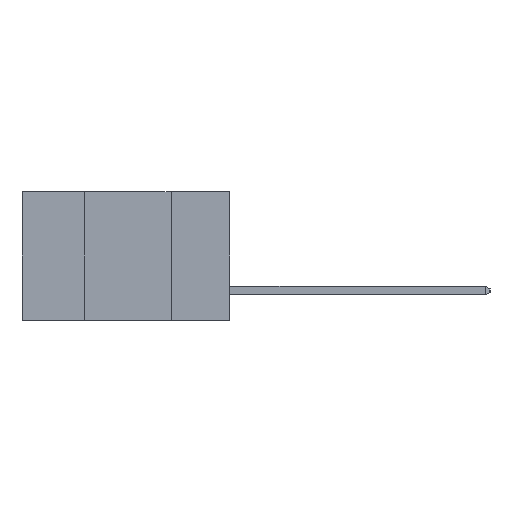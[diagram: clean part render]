
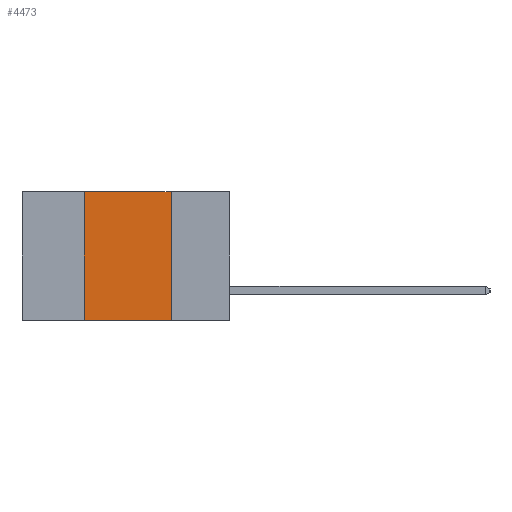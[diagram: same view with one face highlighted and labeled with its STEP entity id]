
A CAD part, left-side view. The second image highlights one B-rep face of the part: STEP entity #4473.
In plain terms, the highlighted planar face has unit normal (-1, 0, 0).
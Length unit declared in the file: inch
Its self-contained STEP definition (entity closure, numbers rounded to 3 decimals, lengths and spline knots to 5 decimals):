
#87 = CARTESIAN_POINT ( 'NONE',  ( 0., 0.6, 0. ) ) ;
#470 = DIRECTION ( 'NONE',  ( 1., 0., 0. ) ) ;
#534 = DIRECTION ( 'NONE',  ( 0., 0., -1. ) ) ;
#756 = EDGE_CURVE ( 'NONE', #3559, #2636, #8635, .T. ) ;
#881 = VERTEX_POINT ( 'NONE', #5766 ) ;
#1066 = EDGE_LOOP ( 'NONE', ( #6810, #4870, #7069, #7345 ) ) ;
#1319 = PLANE ( 'NONE',  #10908 ) ;
#1651 = CARTESIAN_POINT ( 'NONE',  ( 0., 0.17, -0.37 ) ) ;
#1844 = CARTESIAN_POINT ( 'NONE',  ( 0., 0.6, -0.37 ) ) ;
#1990 = EDGE_CURVE ( 'NONE', #881, #3559, #8235, .T. ) ;
#2378 = CARTESIAN_POINT ( 'NONE',  ( 0., 0.17, 0. ) ) ;
#2571 = CARTESIAN_POINT ( 'NONE',  ( 0., 0.6, 0. ) ) ;
#2636 = VERTEX_POINT ( 'NONE', #2378 ) ;
#2643 = CARTESIAN_POINT ( 'NONE',  ( 0., 0.17, -0.37 ) ) ;
#3559 = VERTEX_POINT ( 'NONE', #5365 ) ;
#3586 = DIRECTION ( 'NONE',  ( 0., -1., 0. ) ) ;
#4473 = ADVANCED_FACE ( 'NONE', ( #8556 ), #1319, .F. ) ;
#4870 = ORIENTED_EDGE ( 'NONE', *, *, #756, .F. ) ;
#5365 = CARTESIAN_POINT ( 'NONE',  ( 0., 0.42, 0. ) ) ;
#5766 = CARTESIAN_POINT ( 'NONE',  ( 0., 0.42, -0.37 ) ) ;
#6008 = VECTOR ( 'NONE', #7766, 39.37008 ) ;
#6066 = VERTEX_POINT ( 'NONE', #1651 ) ;
#6188 = DIRECTION ( 'NONE',  ( 0., -1., 0. ) ) ;
#6428 = VECTOR ( 'NONE', #3586, 39.37008 ) ;
#6619 = LINE ( 'NONE', #1844, #10853 ) ;
#6810 = ORIENTED_EDGE ( 'NONE', *, *, #9561, .F. ) ;
#7069 = ORIENTED_EDGE ( 'NONE', *, *, #1990, .F. ) ;
#7345 = ORIENTED_EDGE ( 'NONE', *, *, #9023, .T. ) ;
#7721 = CARTESIAN_POINT ( 'NONE',  ( 0., 0.42, -0.37 ) ) ;
#7737 = DIRECTION ( 'NONE',  ( 0., 0., -1. ) ) ;
#7766 = DIRECTION ( 'NONE',  ( 0., 0., 1. ) ) ;
#7783 = LINE ( 'NONE', #2643, #9677 ) ;
#8235 = LINE ( 'NONE', #7721, #6008 ) ;
#8556 = FACE_OUTER_BOUND ( 'NONE', #1066, .T. ) ;
#8635 = LINE ( 'NONE', #2571, #6428 ) ;
#9023 = EDGE_CURVE ( 'NONE', #881, #6066, #6619, .T. ) ;
#9561 = EDGE_CURVE ( 'NONE', #2636, #6066, #7783, .T. ) ;
#9677 = VECTOR ( 'NONE', #7737, 39.37008 ) ;
#10853 = VECTOR ( 'NONE', #6188, 39.37008 ) ;
#10908 = AXIS2_PLACEMENT_3D ( 'NONE', #87, #470, #534 ) ;
